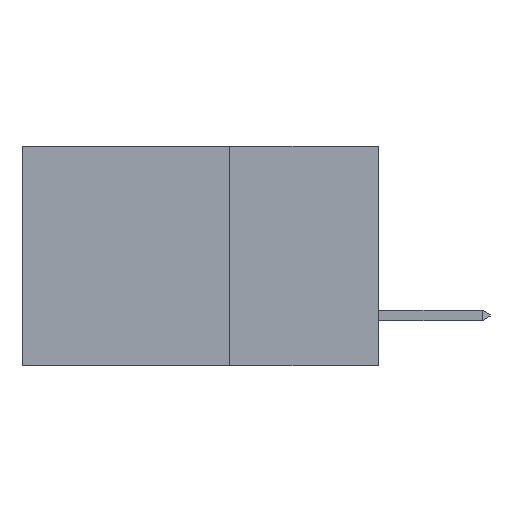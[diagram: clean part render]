
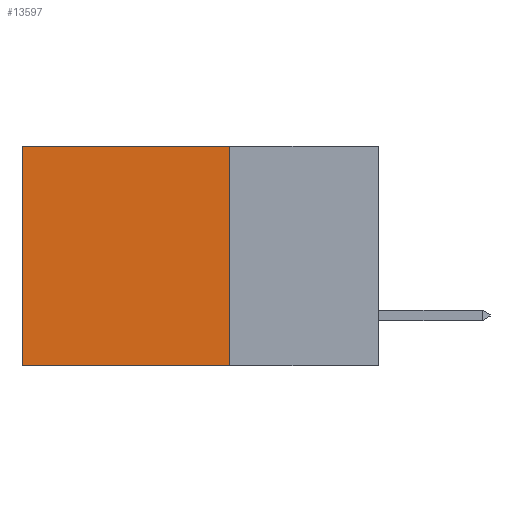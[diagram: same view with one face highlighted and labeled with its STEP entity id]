
A CAD part, left-side view. The second image highlights one B-rep face of the part: STEP entity #13597.
In plain terms, the highlighted planar face has unit normal (-1, 0, 0).
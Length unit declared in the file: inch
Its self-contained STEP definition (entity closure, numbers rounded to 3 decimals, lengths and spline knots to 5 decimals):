
#345 = ORIENTED_EDGE ( 'NONE', *, *, #3203, .T. ) ;
#461 = DIRECTION ( 'NONE',  ( 0., 0., -1. ) ) ;
#662 = CARTESIAN_POINT ( 'NONE',  ( 0.298, 0.25, 0. ) ) ;
#767 = ORIENTED_EDGE ( 'NONE', *, *, #4591, .T. ) ;
#1002 = FACE_OUTER_BOUND ( 'NONE', #14205, .T. ) ;
#1441 = VERTEX_POINT ( 'NONE', #8137 ) ;
#1764 = ORIENTED_EDGE ( 'NONE', *, *, #13516, .F. ) ;
#1831 = DIRECTION ( 'NONE',  ( 0., 0., -1. ) ) ;
#2566 = DIRECTION ( 'NONE',  ( 0., 1., 0. ) ) ;
#3203 = EDGE_CURVE ( 'NONE', #1441, #11203, #7750, .T. ) ;
#3748 = DIRECTION ( 'NONE',  ( 1., 0., 0. ) ) ;
#4591 = EDGE_CURVE ( 'NONE', #9658, #1441, #11615, .T. ) ;
#7750 = LINE ( 'NONE', #10124, #10411 ) ;
#8137 = CARTESIAN_POINT ( 'NONE',  ( 0.298, 0.6, 0. ) ) ;
#8283 = DIRECTION ( 'NONE',  ( 0., 1., 0. ) ) ;
#8383 = PLANE ( 'NONE',  #11626 ) ;
#8735 = VERTEX_POINT ( 'NONE', #9712 ) ;
#9658 = VERTEX_POINT ( 'NONE', #11295 ) ;
#9712 = CARTESIAN_POINT ( 'NONE',  ( 0.298, 0.25, -0.37 ) ) ;
#10124 = CARTESIAN_POINT ( 'NONE',  ( 0.298, 0.6, 0. ) ) ;
#10411 = VECTOR ( 'NONE', #461, 39.37008 ) ;
#10639 = CARTESIAN_POINT ( 'NONE',  ( 0.298, 0.25, 0. ) ) ;
#10711 = CARTESIAN_POINT ( 'NONE',  ( 0.298, 0.25, 0. ) ) ;
#10714 = EDGE_CURVE ( 'NONE', #9658, #8735, #13971, .T. ) ;
#10907 = CARTESIAN_POINT ( 'NONE',  ( 0.298, 0.6, -0.37 ) ) ;
#11203 = VERTEX_POINT ( 'NONE', #10907 ) ;
#11295 = CARTESIAN_POINT ( 'NONE',  ( 0.298, 0.25, 0. ) ) ;
#11311 = LINE ( 'NONE', #13802, #13880 ) ;
#11615 = LINE ( 'NONE', #10711, #14521 ) ;
#11626 = AXIS2_PLACEMENT_3D ( 'NONE', #10639, #3748, #11710 ) ;
#11710 = DIRECTION ( 'NONE',  ( 0., 0., -1. ) ) ;
#13292 = VECTOR ( 'NONE', #1831, 39.37008 ) ;
#13293 = ORIENTED_EDGE ( 'NONE', *, *, #10714, .F. ) ;
#13516 = EDGE_CURVE ( 'NONE', #8735, #11203, #11311, .T. ) ;
#13597 = ADVANCED_FACE ( 'NONE', ( #1002 ), #8383, .F. ) ;
#13802 = CARTESIAN_POINT ( 'NONE',  ( 0.298, 0.25, -0.37 ) ) ;
#13880 = VECTOR ( 'NONE', #8283, 39.37008 ) ;
#13971 = LINE ( 'NONE', #662, #13292 ) ;
#14205 = EDGE_LOOP ( 'NONE', ( #345, #1764, #13293, #767 ) ) ;
#14521 = VECTOR ( 'NONE', #2566, 39.37008 ) ;
